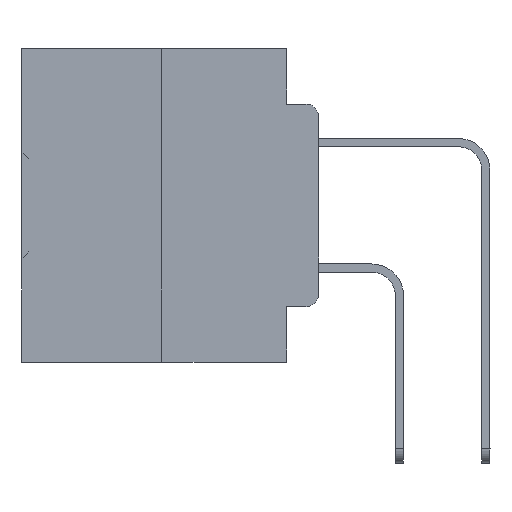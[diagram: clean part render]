
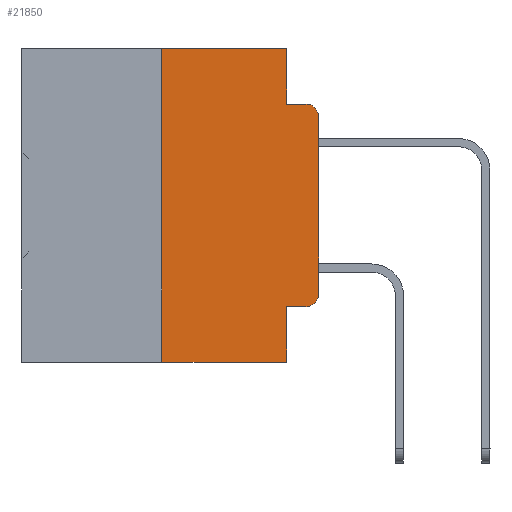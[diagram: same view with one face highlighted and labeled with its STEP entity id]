
A CAD part, left-side view. The second image highlights one B-rep face of the part: STEP entity #21850.
In plain terms, the highlighted planar face has unit normal (-1, 0, 0).
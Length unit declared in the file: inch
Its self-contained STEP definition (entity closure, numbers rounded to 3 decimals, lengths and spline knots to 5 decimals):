
#199 = LINE ( 'NONE', #10136, #17981 ) ;
#365 = ORIENTED_EDGE ( 'NONE', *, *, #21300, .T. ) ;
#707 = EDGE_CURVE ( 'NONE', #8627, #9175, #14168, .T. ) ;
#1015 = VECTOR ( 'NONE', #16156, 39.37008 ) ;
#1078 = DIRECTION ( 'NONE',  ( 0., 0., -1. ) ) ;
#1481 = CARTESIAN_POINT ( 'NONE',  ( 0., 0.02, -0.1085 ) ) ;
#2519 = LINE ( 'NONE', #27585, #12157 ) ;
#2858 = CARTESIAN_POINT ( 'NONE',  ( 0., 0.051, -0.4115 ) ) ;
#3031 = CARTESIAN_POINT ( 'NONE',  ( 0., 0.051, -0.5 ) ) ;
#3486 = CARTESIAN_POINT ( 'NONE',  ( 0., 0.051, -0.0885 ) ) ;
#3966 = CARTESIAN_POINT ( 'NONE',  ( 0., 0.051, -0.0885 ) ) ;
#4392 = EDGE_CURVE ( 'NONE', #8335, #19261, #4491, .T. ) ;
#4491 = CIRCLE ( 'NONE', #12257, 0.02 ) ;
#4702 = LINE ( 'NONE', #13820, #9486 ) ;
#4722 = VERTEX_POINT ( 'NONE', #3486 ) ;
#4832 = CIRCLE ( 'NONE', #9992, 0.02 ) ;
#4953 = VERTEX_POINT ( 'NONE', #11378 ) ;
#4967 = DIRECTION ( 'NONE',  ( 0., -1., 0. ) ) ;
#5729 = ORIENTED_EDGE ( 'NONE', *, *, #23456, .T. ) ;
#6790 = LINE ( 'NONE', #3966, #1015 ) ;
#7019 = ORIENTED_EDGE ( 'NONE', *, *, #33613, .T. ) ;
#7576 = DIRECTION ( 'NONE',  ( -1., 0., 0. ) ) ;
#8088 = DIRECTION ( 'NONE',  ( 0., 0., -1. ) ) ;
#8335 = VERTEX_POINT ( 'NONE', #21389 ) ;
#8627 = VERTEX_POINT ( 'NONE', #26455 ) ;
#9175 = VERTEX_POINT ( 'NONE', #22728 ) ;
#9486 = VECTOR ( 'NONE', #19564, 39.37008 ) ;
#9992 = AXIS2_PLACEMENT_3D ( 'NONE', #25131, #32091, #1078 ) ;
#10136 = CARTESIAN_POINT ( 'NONE',  ( 0., 0.473, -0.5 ) ) ;
#10206 = LINE ( 'NONE', #38449, #15506 ) ;
#11378 = CARTESIAN_POINT ( 'NONE',  ( 0., 0., -0.3915 ) ) ;
#11718 = EDGE_CURVE ( 'NONE', #28281, #39605, #14278, .T. ) ;
#12157 = VECTOR ( 'NONE', #20856, 39.37008 ) ;
#12231 = ORIENTED_EDGE ( 'NONE', *, *, #4392, .T. ) ;
#12257 = AXIS2_PLACEMENT_3D ( 'NONE', #1481, #7576, #35161 ) ;
#12580 = DIRECTION ( 'NONE',  ( 0., -1., 0. ) ) ;
#13641 = CARTESIAN_POINT ( 'NONE',  ( 0., 0.02, -0.4115 ) ) ;
#13766 = DIRECTION ( 'NONE',  ( 0., 0., 1. ) ) ;
#13820 = CARTESIAN_POINT ( 'NONE',  ( 0., 0.051, 0. ) ) ;
#14168 = LINE ( 'NONE', #19692, #36199 ) ;
#14268 = EDGE_CURVE ( 'NONE', #34377, #4722, #4702, .T. ) ;
#14278 = LINE ( 'NONE', #14686, #38627 ) ;
#14686 = CARTESIAN_POINT ( 'NONE',  ( 0., 0.051, 0. ) ) ;
#15506 = VECTOR ( 'NONE', #34757, 39.37008 ) ;
#15849 = VECTOR ( 'NONE', #4967, 39.37008 ) ;
#16156 = DIRECTION ( 'NONE',  ( 0., -1., 0. ) ) ;
#17981 = VECTOR ( 'NONE', #12580, 39.37008 ) ;
#18259 = CARTESIAN_POINT ( 'NONE',  ( 0., 0.02, -0.0885 ) ) ;
#19261 = VERTEX_POINT ( 'NONE', #18259 ) ;
#19530 = ORIENTED_EDGE ( 'NONE', *, *, #22549, .F. ) ;
#19564 = DIRECTION ( 'NONE',  ( 0., 0., -1. ) ) ;
#19692 = CARTESIAN_POINT ( 'NONE',  ( 0., 0.25, 0. ) ) ;
#20289 = ORIENTED_EDGE ( 'NONE', *, *, #14268, .F. ) ;
#20856 = DIRECTION ( 'NONE',  ( 0., -1., 0. ) ) ;
#21300 = EDGE_CURVE ( 'NONE', #30494, #4953, #4832, .T. ) ;
#21389 = CARTESIAN_POINT ( 'NONE',  ( 0., 0., -0.1085 ) ) ;
#21850 = ADVANCED_FACE ( 'NONE', ( #26447 ), #38959, .F. ) ;
#22549 = EDGE_CURVE ( 'NONE', #4722, #19261, #6790, .T. ) ;
#22728 = CARTESIAN_POINT ( 'NONE',  ( 0., 0.25, 0. ) ) ;
#22902 = ORIENTED_EDGE ( 'NONE', *, *, #37324, .F. ) ;
#23255 = ORIENTED_EDGE ( 'NONE', *, *, #707, .F. ) ;
#23456 = EDGE_CURVE ( 'NONE', #8627, #39605, #199, .T. ) ;
#25131 = CARTESIAN_POINT ( 'NONE',  ( 0., 0.02, -0.3915 ) ) ;
#26217 = CARTESIAN_POINT ( 'NONE',  ( 0., 0.051, 0. ) ) ;
#26447 = FACE_OUTER_BOUND ( 'NONE', #29977, .T. ) ;
#26455 = CARTESIAN_POINT ( 'NONE',  ( 0., 0.25, -0.5 ) ) ;
#26533 = DIRECTION ( 'NONE',  ( 0., 0., -1. ) ) ;
#26646 = ORIENTED_EDGE ( 'NONE', *, *, #27332, .T. ) ;
#26856 = DIRECTION ( 'NONE',  ( 1., 0., 0. ) ) ;
#27002 = CARTESIAN_POINT ( 'NONE',  ( 0., 0.051, -0.4115 ) ) ;
#27332 = EDGE_CURVE ( 'NONE', #4953, #8335, #10206, .T. ) ;
#27585 = CARTESIAN_POINT ( 'NONE',  ( 0., 0.473, 0. ) ) ;
#28281 = VERTEX_POINT ( 'NONE', #27002 ) ;
#29977 = EDGE_LOOP ( 'NONE', ( #26646, #12231, #19530, #20289, #22902, #23255, #5729, #38963, #7019, #365 ) ) ;
#30494 = VERTEX_POINT ( 'NONE', #13641 ) ;
#32091 = DIRECTION ( 'NONE',  ( -1., 0., 0. ) ) ;
#33613 = EDGE_CURVE ( 'NONE', #28281, #30494, #40247, .T. ) ;
#34377 = VERTEX_POINT ( 'NONE', #26217 ) ;
#34757 = DIRECTION ( 'NONE',  ( 0., 0., 1. ) ) ;
#35161 = DIRECTION ( 'NONE',  ( 0., 0., -1. ) ) ;
#35470 = CARTESIAN_POINT ( 'NONE',  ( 0., 0.473, 0. ) ) ;
#36199 = VECTOR ( 'NONE', #13766, 39.37008 ) ;
#37324 = EDGE_CURVE ( 'NONE', #9175, #34377, #2519, .T. ) ;
#38151 = AXIS2_PLACEMENT_3D ( 'NONE', #35470, #26856, #8088 ) ;
#38449 = CARTESIAN_POINT ( 'NONE',  ( 0., 0., 0. ) ) ;
#38627 = VECTOR ( 'NONE', #26533, 39.37008 ) ;
#38959 = PLANE ( 'NONE',  #38151 ) ;
#38963 = ORIENTED_EDGE ( 'NONE', *, *, #11718, .F. ) ;
#39605 = VERTEX_POINT ( 'NONE', #3031 ) ;
#40247 = LINE ( 'NONE', #2858, #15849 ) ;
